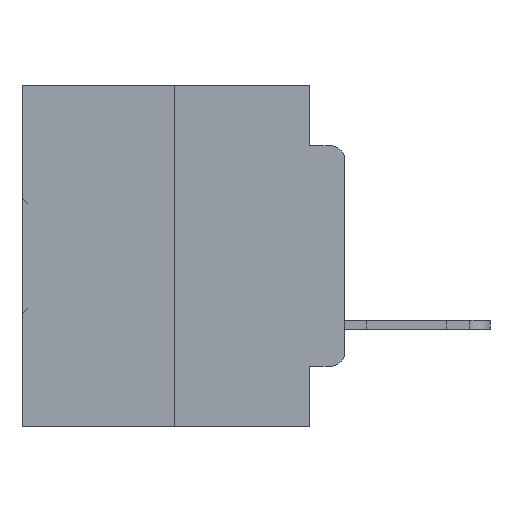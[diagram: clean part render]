
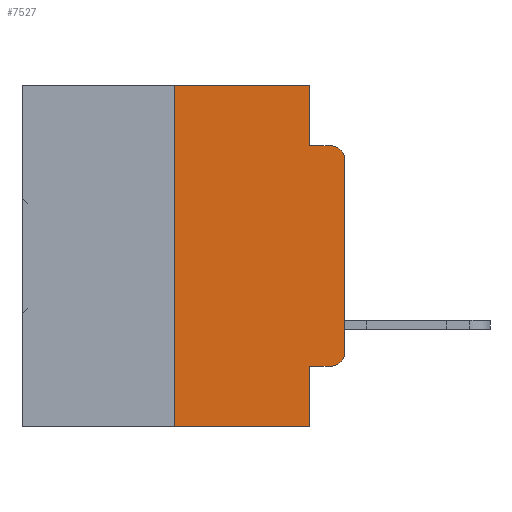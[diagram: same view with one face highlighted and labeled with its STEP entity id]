
A CAD part, left-side view. The second image highlights one B-rep face of the part: STEP entity #7527.
In plain terms, the highlighted planar face has unit normal (-1, 0, 0).
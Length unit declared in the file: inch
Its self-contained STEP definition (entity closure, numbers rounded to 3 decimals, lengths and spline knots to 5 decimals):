
#703 = CARTESIAN_POINT ( 'NONE',  ( 0., 0.051, 0. ) ) ;
#1095 = DIRECTION ( 'NONE',  ( 0., 0., 1. ) ) ;
#1771 = LINE ( 'NONE', #21396, #9043 ) ;
#1854 = CARTESIAN_POINT ( 'NONE',  ( 0., 0.25, -0.5 ) ) ;
#2017 = EDGE_CURVE ( 'NONE', #26853, #22794, #1771, .T. ) ;
#2069 = CARTESIAN_POINT ( 'NONE',  ( 0., 0.02, -0.3915 ) ) ;
#2263 = VERTEX_POINT ( 'NONE', #29762 ) ;
#3027 = VERTEX_POINT ( 'NONE', #22421 ) ;
#3243 = EDGE_CURVE ( 'NONE', #10468, #32382, #35091, .T. ) ;
#4811 = LINE ( 'NONE', #15415, #19099 ) ;
#4917 = ORIENTED_EDGE ( 'NONE', *, *, #28217, .F. ) ;
#5150 = DIRECTION ( 'NONE',  ( 0., 0., -1. ) ) ;
#5642 = VERTEX_POINT ( 'NONE', #19348 ) ;
#5983 = DIRECTION ( 'NONE',  ( 0., 0., -1. ) ) ;
#6096 = AXIS2_PLACEMENT_3D ( 'NONE', #2069, #21965, #5150 ) ;
#6508 = ORIENTED_EDGE ( 'NONE', *, *, #25816, .T. ) ;
#6810 = DIRECTION ( 'NONE',  ( 0., -1., 0. ) ) ;
#6928 = ORIENTED_EDGE ( 'NONE', *, *, #17584, .T. ) ;
#7527 = ADVANCED_FACE ( 'NONE', ( #35580 ), #20959, .F. ) ;
#7614 = EDGE_LOOP ( 'NONE', ( #6508, #16619, #24695, #24847, #25111, #29639, #30555, #4917, #15093, #6928 ) ) ;
#8463 = VERTEX_POINT ( 'NONE', #19033 ) ;
#9043 = VECTOR ( 'NONE', #21196, 39.37008 ) ;
#9525 = DIRECTION ( 'NONE',  ( 0., -1., 0. ) ) ;
#9756 = VECTOR ( 'NONE', #9525, 39.37008 ) ;
#10084 = DIRECTION ( 'NONE',  ( 0., 0., 1. ) ) ;
#10364 = CIRCLE ( 'NONE', #35006, 0.02 ) ;
#10468 = VERTEX_POINT ( 'NONE', #703 ) ;
#11915 = DIRECTION ( 'NONE',  ( 0., -1., 0. ) ) ;
#12307 = VERTEX_POINT ( 'NONE', #33578 ) ;
#14351 = VECTOR ( 'NONE', #20091, 39.37008 ) ;
#15093 = ORIENTED_EDGE ( 'NONE', *, *, #24721, .T. ) ;
#15144 = EDGE_CURVE ( 'NONE', #32382, #8463, #4811, .T. ) ;
#15201 = LINE ( 'NONE', #33807, #20487 ) ;
#15415 = CARTESIAN_POINT ( 'NONE',  ( 0., 0.051, -0.0885 ) ) ;
#15849 = CARTESIAN_POINT ( 'NONE',  ( 0., 0., 0. ) ) ;
#16619 = ORIENTED_EDGE ( 'NONE', *, *, #24041, .T. ) ;
#16838 = CARTESIAN_POINT ( 'NONE',  ( 0., 0.051, -0.0885 ) ) ;
#17453 = CARTESIAN_POINT ( 'NONE',  ( 0., 0.02, -0.1085 ) ) ;
#17584 = EDGE_CURVE ( 'NONE', #12307, #25403, #30321, .T. ) ;
#18527 = EDGE_CURVE ( 'NONE', #5642, #10468, #30264, .T. ) ;
#19033 = CARTESIAN_POINT ( 'NONE',  ( 0., 0.02, -0.0885 ) ) ;
#19099 = VECTOR ( 'NONE', #6810, 39.37008 ) ;
#19348 = CARTESIAN_POINT ( 'NONE',  ( 0., 0.25, 0. ) ) ;
#19950 = CARTESIAN_POINT ( 'NONE',  ( 0., 0.051, 0. ) ) ;
#20025 = DIRECTION ( 'NONE',  ( 0., 0., -1. ) ) ;
#20090 = DIRECTION ( 'NONE',  ( 0., 0., -1. ) ) ;
#20091 = DIRECTION ( 'NONE',  ( 0., 0., -1. ) ) ;
#20379 = CARTESIAN_POINT ( 'NONE',  ( 0., 0.051, 0. ) ) ;
#20450 = LINE ( 'NONE', #33056, #34283 ) ;
#20487 = VECTOR ( 'NONE', #10084, 39.37008 ) ;
#20715 = DIRECTION ( 'NONE',  ( 1., 0., 0. ) ) ;
#20959 = PLANE ( 'NONE',  #28534 ) ;
#21196 = DIRECTION ( 'NONE',  ( 0., -1., 0. ) ) ;
#21247 = VECTOR ( 'NONE', #1095, 39.37008 ) ;
#21396 = CARTESIAN_POINT ( 'NONE',  ( 0., 0.473, -0.5 ) ) ;
#21575 = CARTESIAN_POINT ( 'NONE',  ( 0., 0.473, 0. ) ) ;
#21965 = DIRECTION ( 'NONE',  ( -1., 0., 0. ) ) ;
#22421 = CARTESIAN_POINT ( 'NONE',  ( 0., 0., -0.1085 ) ) ;
#22791 = VECTOR ( 'NONE', #5983, 39.37008 ) ;
#22794 = VERTEX_POINT ( 'NONE', #34643 ) ;
#24041 = EDGE_CURVE ( 'NONE', #3027, #8463, #10364, .T. ) ;
#24695 = ORIENTED_EDGE ( 'NONE', *, *, #15144, .F. ) ;
#24721 = EDGE_CURVE ( 'NONE', #2263, #12307, #20450, .T. ) ;
#24847 = ORIENTED_EDGE ( 'NONE', *, *, #3243, .F. ) ;
#25111 = ORIENTED_EDGE ( 'NONE', *, *, #18527, .F. ) ;
#25403 = VERTEX_POINT ( 'NONE', #35243 ) ;
#25816 = EDGE_CURVE ( 'NONE', #25403, #3027, #27519, .T. ) ;
#26853 = VERTEX_POINT ( 'NONE', #1854 ) ;
#27519 = LINE ( 'NONE', #15849, #21247 ) ;
#28217 = EDGE_CURVE ( 'NONE', #2263, #22794, #30548, .T. ) ;
#28534 = AXIS2_PLACEMENT_3D ( 'NONE', #21575, #20715, #20090 ) ;
#29639 = ORIENTED_EDGE ( 'NONE', *, *, #34937, .F. ) ;
#29762 = CARTESIAN_POINT ( 'NONE',  ( 0., 0.051, -0.4115 ) ) ;
#30264 = LINE ( 'NONE', #30822, #9756 ) ;
#30321 = CIRCLE ( 'NONE', #6096, 0.02 ) ;
#30548 = LINE ( 'NONE', #19950, #22791 ) ;
#30555 = ORIENTED_EDGE ( 'NONE', *, *, #2017, .T. ) ;
#30822 = CARTESIAN_POINT ( 'NONE',  ( 0., 0.473, 0. ) ) ;
#32382 = VERTEX_POINT ( 'NONE', #16838 ) ;
#33056 = CARTESIAN_POINT ( 'NONE',  ( 0., 0.051, -0.4115 ) ) ;
#33578 = CARTESIAN_POINT ( 'NONE',  ( 0., 0.02, -0.4115 ) ) ;
#33807 = CARTESIAN_POINT ( 'NONE',  ( 0., 0.25, 0. ) ) ;
#34283 = VECTOR ( 'NONE', #11915, 39.37008 ) ;
#34643 = CARTESIAN_POINT ( 'NONE',  ( 0., 0.051, -0.5 ) ) ;
#34937 = EDGE_CURVE ( 'NONE', #26853, #5642, #15201, .T. ) ;
#35006 = AXIS2_PLACEMENT_3D ( 'NONE', #17453, #35524, #20025 ) ;
#35091 = LINE ( 'NONE', #20379, #14351 ) ;
#35243 = CARTESIAN_POINT ( 'NONE',  ( 0., 0., -0.3915 ) ) ;
#35524 = DIRECTION ( 'NONE',  ( -1., 0., 0. ) ) ;
#35580 = FACE_OUTER_BOUND ( 'NONE', #7614, .T. ) ;
